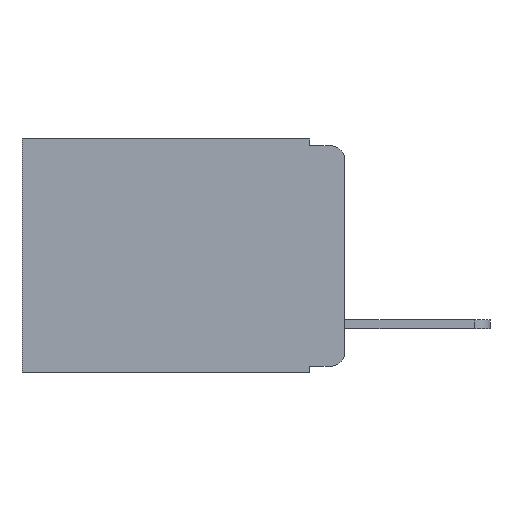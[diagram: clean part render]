
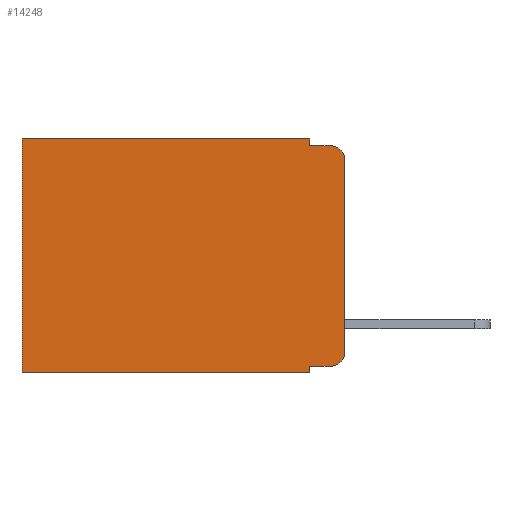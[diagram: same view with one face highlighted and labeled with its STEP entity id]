
A CAD part, left-side view. The second image highlights one B-rep face of the part: STEP entity #14248.
In plain terms, the highlighted planar face has unit normal (-1, 0, 0).
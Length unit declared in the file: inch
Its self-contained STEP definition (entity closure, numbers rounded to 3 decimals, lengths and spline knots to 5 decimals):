
#246 = LINE ( 'NONE', #13871, #17514 ) ;
#291 = EDGE_CURVE ( 'NONE', #21068, #723, #19403, .T. ) ;
#459 = CARTESIAN_POINT ( 'NONE',  ( 0.298, 0.051, -0.333 ) ) ;
#575 = CIRCLE ( 'NONE', #13799, 0.02 ) ;
#723 = VERTEX_POINT ( 'NONE', #4457 ) ;
#802 = ORIENTED_EDGE ( 'NONE', *, *, #6645, .T. ) ;
#897 = CARTESIAN_POINT ( 'NONE',  ( 0.298, 0.051, 0. ) ) ;
#1078 = ORIENTED_EDGE ( 'NONE', *, *, #3789, .T. ) ;
#1375 = DIRECTION ( 'NONE',  ( 0., -1., 0. ) ) ;
#1475 = CARTESIAN_POINT ( 'NONE',  ( 0.298, 0.02, -0.01 ) ) ;
#1512 = DIRECTION ( 'NONE',  ( 1., 0., 0. ) ) ;
#1912 = CARTESIAN_POINT ( 'NONE',  ( 0.298, 0.02, -0.333 ) ) ;
#2261 = LINE ( 'NONE', #5528, #19288 ) ;
#2374 = CARTESIAN_POINT ( 'NONE',  ( 0.298, 0., -0.03 ) ) ;
#2404 = CARTESIAN_POINT ( 'NONE',  ( 0.298, 0.051, 0. ) ) ;
#2422 = VERTEX_POINT ( 'NONE', #1475 ) ;
#2716 = EDGE_CURVE ( 'NONE', #4688, #16007, #17828, .T. ) ;
#2752 = DIRECTION ( 'NONE',  ( 0., -1., 0. ) ) ;
#3155 = CARTESIAN_POINT ( 'NONE',  ( 0.298, 0.051, -0.333 ) ) ;
#3174 = DIRECTION ( 'NONE',  ( -1., 0., 0. ) ) ;
#3378 = ORIENTED_EDGE ( 'NONE', *, *, #9495, .F. ) ;
#3727 = DIRECTION ( 'NONE',  ( 0., 1., 0. ) ) ;
#3789 = EDGE_CURVE ( 'NONE', #4688, #4423, #12522, .T. ) ;
#4423 = VERTEX_POINT ( 'NONE', #1912 ) ;
#4432 = ORIENTED_EDGE ( 'NONE', *, *, #16001, .T. ) ;
#4457 = CARTESIAN_POINT ( 'NONE',  ( 0.298, 0.473, -0.343 ) ) ;
#4688 = VERTEX_POINT ( 'NONE', #3155 ) ;
#5075 = EDGE_CURVE ( 'NONE', #16916, #14132, #246, .T. ) ;
#5080 = ORIENTED_EDGE ( 'NONE', *, *, #2716, .F. ) ;
#5528 = CARTESIAN_POINT ( 'NONE',  ( 0.298, 0., 0. ) ) ;
#5565 = ORIENTED_EDGE ( 'NONE', *, *, #9021, .F. ) ;
#5656 = ORIENTED_EDGE ( 'NONE', *, *, #20453, .F. ) ;
#6636 = CARTESIAN_POINT ( 'NONE',  ( 0.298, 0.051, -0.343 ) ) ;
#6645 = EDGE_CURVE ( 'NONE', #4423, #12988, #7979, .T. ) ;
#6960 = CARTESIAN_POINT ( 'NONE',  ( 0.298, 0.02, -0.03 ) ) ;
#7399 = AXIS2_PLACEMENT_3D ( 'NONE', #13131, #3174, #14750 ) ;
#7979 = CIRCLE ( 'NONE', #7399, 0.02 ) ;
#7982 = VECTOR ( 'NONE', #21277, 39.37008 ) ;
#8166 = DIRECTION ( 'NONE',  ( 0., 0., -1. ) ) ;
#8506 = LINE ( 'NONE', #19676, #7982 ) ;
#8595 = DIRECTION ( 'NONE',  ( 0., 0., -1. ) ) ;
#8760 = ORIENTED_EDGE ( 'NONE', *, *, #19124, .T. ) ;
#9021 = EDGE_CURVE ( 'NONE', #16007, #723, #17414, .T. ) ;
#9087 = EDGE_LOOP ( 'NONE', ( #5656, #8760, #3378, #19266, #4432, #21020, #5565, #5080, #1078, #802 ) ) ;
#9186 = VECTOR ( 'NONE', #19849, 39.37008 ) ;
#9495 = EDGE_CURVE ( 'NONE', #14132, #2422, #20668, .T. ) ;
#9742 = CARTESIAN_POINT ( 'NONE',  ( 0.298, 0., -0.313 ) ) ;
#11281 = CARTESIAN_POINT ( 'NONE',  ( 0.298, 0.051, -0.01 ) ) ;
#11483 = VECTOR ( 'NONE', #2752, 39.37008 ) ;
#11644 = CARTESIAN_POINT ( 'NONE',  ( 0.298, 0., 0. ) ) ;
#12522 = LINE ( 'NONE', #459, #11483 ) ;
#12988 = VERTEX_POINT ( 'NONE', #9742 ) ;
#13131 = CARTESIAN_POINT ( 'NONE',  ( 0.298, 0.02, -0.313 ) ) ;
#13266 = DIRECTION ( 'NONE',  ( 0., 0., -1. ) ) ;
#13626 = VECTOR ( 'NONE', #3727, 39.37008 ) ;
#13700 = FACE_OUTER_BOUND ( 'NONE', #9087, .T. ) ;
#13799 = AXIS2_PLACEMENT_3D ( 'NONE', #6960, #18352, #8595 ) ;
#13871 = CARTESIAN_POINT ( 'NONE',  ( 0.298, 0.051, 0. ) ) ;
#14132 = VERTEX_POINT ( 'NONE', #11281 ) ;
#14248 = ADVANCED_FACE ( 'NONE', ( #13700 ), #16451, .F. ) ;
#14553 = CARTESIAN_POINT ( 'NONE',  ( 0.298, 0.473, 0. ) ) ;
#14647 = AXIS2_PLACEMENT_3D ( 'NONE', #11644, #1512, #13266 ) ;
#14693 = CARTESIAN_POINT ( 'NONE',  ( 0.298, 0.051, -0.01 ) ) ;
#14750 = DIRECTION ( 'NONE',  ( 0., 0., -1. ) ) ;
#15129 = VECTOR ( 'NONE', #16855, 39.37008 ) ;
#15370 = DIRECTION ( 'NONE',  ( 0., 0., -1. ) ) ;
#16001 = EDGE_CURVE ( 'NONE', #16916, #21068, #8506, .T. ) ;
#16007 = VERTEX_POINT ( 'NONE', #6636 ) ;
#16311 = VERTEX_POINT ( 'NONE', #2374 ) ;
#16418 = CARTESIAN_POINT ( 'NONE',  ( 0.298, 0.473, 0. ) ) ;
#16451 = PLANE ( 'NONE',  #14647 ) ;
#16855 = DIRECTION ( 'NONE',  ( 0., 0., -1. ) ) ;
#16897 = CARTESIAN_POINT ( 'NONE',  ( 0.298, 0., -0.343 ) ) ;
#16916 = VERTEX_POINT ( 'NONE', #897 ) ;
#17414 = LINE ( 'NONE', #16897, #13626 ) ;
#17514 = VECTOR ( 'NONE', #8166, 39.37008 ) ;
#17828 = LINE ( 'NONE', #2404, #9186 ) ;
#18352 = DIRECTION ( 'NONE',  ( -1., 0., 0. ) ) ;
#19124 = EDGE_CURVE ( 'NONE', #16311, #2422, #575, .T. ) ;
#19266 = ORIENTED_EDGE ( 'NONE', *, *, #5075, .F. ) ;
#19288 = VECTOR ( 'NONE', #15370, 39.37008 ) ;
#19403 = LINE ( 'NONE', #16418, #15129 ) ;
#19676 = CARTESIAN_POINT ( 'NONE',  ( 0.298, 0., 0. ) ) ;
#19849 = DIRECTION ( 'NONE',  ( 0., 0., -1. ) ) ;
#20165 = VECTOR ( 'NONE', #1375, 39.37008 ) ;
#20453 = EDGE_CURVE ( 'NONE', #16311, #12988, #2261, .T. ) ;
#20668 = LINE ( 'NONE', #14693, #20165 ) ;
#21020 = ORIENTED_EDGE ( 'NONE', *, *, #291, .T. ) ;
#21068 = VERTEX_POINT ( 'NONE', #14553 ) ;
#21277 = DIRECTION ( 'NONE',  ( 0., 1., 0. ) ) ;
